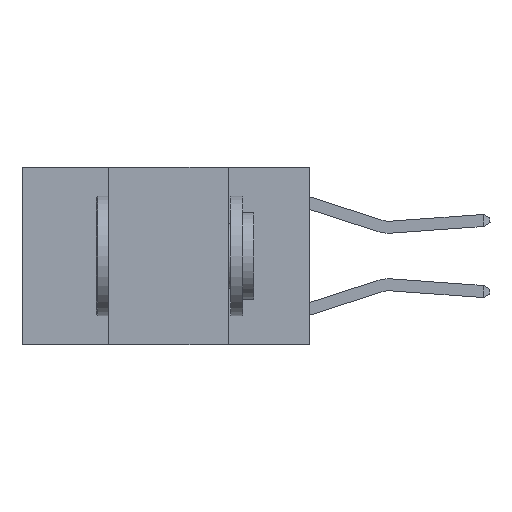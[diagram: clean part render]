
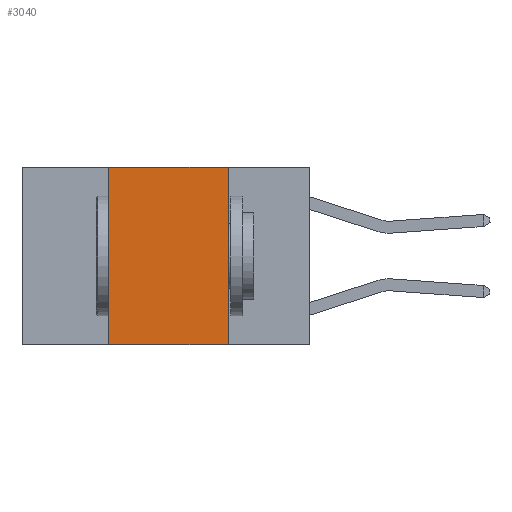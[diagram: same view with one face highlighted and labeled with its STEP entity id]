
A CAD part, left-side view. The second image highlights one B-rep face of the part: STEP entity #3040.
In plain terms, the highlighted planar face has unit normal (-1, 0, 0).
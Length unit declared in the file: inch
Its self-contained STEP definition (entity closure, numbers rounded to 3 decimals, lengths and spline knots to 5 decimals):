
#59 = VECTOR ( 'NONE', #4969, 39.37008 ) ;
#443 = LINE ( 'NONE', #13616, #59 ) ;
#542 = DIRECTION ( 'NONE',  ( 0., 0., -1. ) ) ;
#559 = DIRECTION ( 'NONE',  ( 1., 0., 0. ) ) ;
#661 = CARTESIAN_POINT ( 'NONE',  ( 0., 0.6, 0. ) ) ;
#714 = PLANE ( 'NONE',  #3849 ) ;
#1271 = CARTESIAN_POINT ( 'NONE',  ( 0., 0.6, -0.37 ) ) ;
#1435 = VECTOR ( 'NONE', #11915, 39.37008 ) ;
#1959 = VECTOR ( 'NONE', #12082, 39.37008 ) ;
#2339 = LINE ( 'NONE', #4462, #1959 ) ;
#3040 = ADVANCED_FACE ( 'NONE', ( #5441 ), #714, .F. ) ;
#3849 = AXIS2_PLACEMENT_3D ( 'NONE', #661, #559, #542 ) ;
#3853 = VERTEX_POINT ( 'NONE', #10503 ) ;
#4006 = EDGE_CURVE ( 'NONE', #10531, #4812, #13185, .T. ) ;
#4462 = CARTESIAN_POINT ( 'NONE',  ( 0., 0.17, 0. ) ) ;
#4789 = DIRECTION ( 'NONE',  ( 0., -1., 0. ) ) ;
#4812 = VERTEX_POINT ( 'NONE', #12262 ) ;
#4969 = DIRECTION ( 'NONE',  ( 0., 0., 1. ) ) ;
#5441 = FACE_OUTER_BOUND ( 'NONE', #12622, .T. ) ;
#5511 = ORIENTED_EDGE ( 'NONE', *, *, #5594, .T. ) ;
#5594 = EDGE_CURVE ( 'NONE', #3853, #7876, #8199, .T. ) ;
#6645 = EDGE_CURVE ( 'NONE', #4812, #7876, #2339, .T. ) ;
#7786 = ORIENTED_EDGE ( 'NONE', *, *, #6645, .F. ) ;
#7876 = VERTEX_POINT ( 'NONE', #14203 ) ;
#8132 = EDGE_CURVE ( 'NONE', #3853, #10531, #443, .T. ) ;
#8137 = ORIENTED_EDGE ( 'NONE', *, *, #4006, .F. ) ;
#8199 = LINE ( 'NONE', #1271, #13519 ) ;
#9822 = CARTESIAN_POINT ( 'NONE',  ( 0., 0.42, 0. ) ) ;
#10503 = CARTESIAN_POINT ( 'NONE',  ( 0., 0.42, -0.37 ) ) ;
#10531 = VERTEX_POINT ( 'NONE', #9822 ) ;
#11863 = CARTESIAN_POINT ( 'NONE',  ( 0., 0.6, 0. ) ) ;
#11915 = DIRECTION ( 'NONE',  ( 0., -1., 0. ) ) ;
#12082 = DIRECTION ( 'NONE',  ( 0., 0., -1. ) ) ;
#12262 = CARTESIAN_POINT ( 'NONE',  ( 0., 0.17, 0. ) ) ;
#12622 = EDGE_LOOP ( 'NONE', ( #7786, #8137, #13780, #5511 ) ) ;
#13185 = LINE ( 'NONE', #11863, #1435 ) ;
#13519 = VECTOR ( 'NONE', #4789, 39.37008 ) ;
#13616 = CARTESIAN_POINT ( 'NONE',  ( 0., 0.42, 0. ) ) ;
#13780 = ORIENTED_EDGE ( 'NONE', *, *, #8132, .F. ) ;
#14203 = CARTESIAN_POINT ( 'NONE',  ( 0., 0.17, -0.37 ) ) ;
